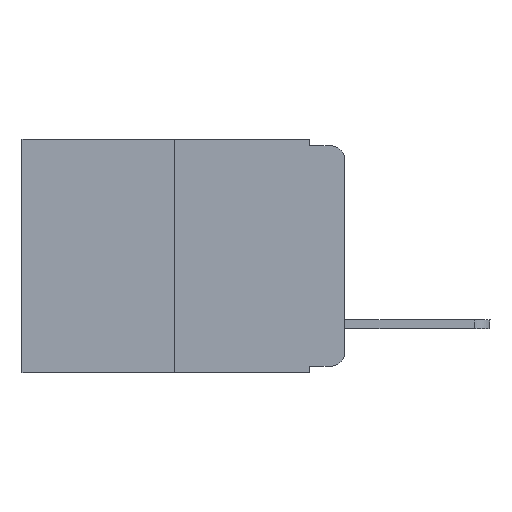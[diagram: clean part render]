
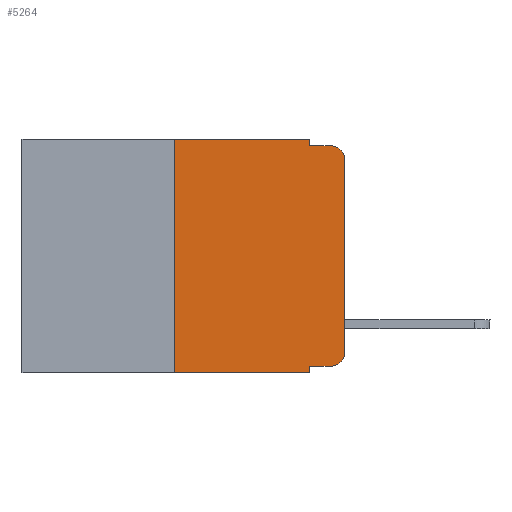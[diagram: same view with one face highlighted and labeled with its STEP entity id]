
A CAD part, left-side view. The second image highlights one B-rep face of the part: STEP entity #5264.
In plain terms, the highlighted planar face has unit normal (-1, 0, 0).
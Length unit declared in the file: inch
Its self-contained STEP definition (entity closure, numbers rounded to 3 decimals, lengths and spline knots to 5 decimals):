
#250 = EDGE_CURVE ( 'NONE', #9479, #11824, #8572, .T. ) ;
#260 = VECTOR ( 'NONE', #2099, 39.37008 ) ;
#417 = ORIENTED_EDGE ( 'NONE', *, *, #2067, .F. ) ;
#451 = EDGE_CURVE ( 'NONE', #14695, #15219, #6794, .T. ) ;
#776 = DIRECTION ( 'NONE',  ( 0., 0., -1. ) ) ;
#1366 = CARTESIAN_POINT ( 'NONE',  ( 0., 0.02, -0.01 ) ) ;
#1381 = EDGE_CURVE ( 'NONE', #6574, #12329, #13996, .T. ) ;
#1649 = LINE ( 'NONE', #4999, #11156 ) ;
#1793 = VECTOR ( 'NONE', #5993, 39.37008 ) ;
#2029 = CARTESIAN_POINT ( 'NONE',  ( 0., 0.051, 0. ) ) ;
#2041 = VECTOR ( 'NONE', #11379, 39.37008 ) ;
#2067 = EDGE_CURVE ( 'NONE', #7945, #11824, #14886, .T. ) ;
#2099 = DIRECTION ( 'NONE',  ( 0., 0., 1. ) ) ;
#2555 = VECTOR ( 'NONE', #5166, 39.37008 ) ;
#2570 = ORIENTED_EDGE ( 'NONE', *, *, #13722, .T. ) ;
#2808 = CARTESIAN_POINT ( 'NONE',  ( 0., 0.25, -0.343 ) ) ;
#2891 = CARTESIAN_POINT ( 'NONE',  ( 0., 0., 0. ) ) ;
#3054 = DIRECTION ( 'NONE',  ( 0., 0., 1. ) ) ;
#3152 = ORIENTED_EDGE ( 'NONE', *, *, #7505, .F. ) ;
#3263 = CARTESIAN_POINT ( 'NONE',  ( 0., 0.473, 0. ) ) ;
#3292 = CARTESIAN_POINT ( 'NONE',  ( 0., 0.051, -0.333 ) ) ;
#3336 = VERTEX_POINT ( 'NONE', #2808 ) ;
#3436 = ORIENTED_EDGE ( 'NONE', *, *, #4660, .F. ) ;
#3578 = AXIS2_PLACEMENT_3D ( 'NONE', #7578, #4042, #12323 ) ;
#3609 = CARTESIAN_POINT ( 'NONE',  ( 0., 0.02, -0.333 ) ) ;
#4042 = DIRECTION ( 'NONE',  ( -1., 0., 0. ) ) ;
#4388 = ORIENTED_EDGE ( 'NONE', *, *, #9475, .T. ) ;
#4435 = PLANE ( 'NONE',  #4990 ) ;
#4517 = LINE ( 'NONE', #5526, #260 ) ;
#4660 = EDGE_CURVE ( 'NONE', #15219, #7945, #6656, .T. ) ;
#4837 = CARTESIAN_POINT ( 'NONE',  ( 0., 0.25, 0. ) ) ;
#4990 = AXIS2_PLACEMENT_3D ( 'NONE', #3263, #12548, #776 ) ;
#4999 = CARTESIAN_POINT ( 'NONE',  ( 0., 0.051, 0. ) ) ;
#5076 = EDGE_LOOP ( 'NONE', ( #2570, #13152, #417, #3436, #9999, #10802, #4388, #3152, #5623, #9858 ) ) ;
#5166 = DIRECTION ( 'NONE',  ( 0., 0., -1. ) ) ;
#5264 = ADVANCED_FACE ( 'NONE', ( #11463 ), #4435, .F. ) ;
#5526 = CARTESIAN_POINT ( 'NONE',  ( 0., 0.25, 0. ) ) ;
#5623 = ORIENTED_EDGE ( 'NONE', *, *, #1381, .T. ) ;
#5993 = DIRECTION ( 'NONE',  ( 0., -1., 0. ) ) ;
#6017 = EDGE_CURVE ( 'NONE', #12329, #7464, #10867, .T. ) ;
#6271 = CARTESIAN_POINT ( 'NONE',  ( 0., 0.051, -0.343 ) ) ;
#6347 = DIRECTION ( 'NONE',  ( 0., 0., -1. ) ) ;
#6574 = VERTEX_POINT ( 'NONE', #7779 ) ;
#6656 = LINE ( 'NONE', #2029, #2555 ) ;
#6794 = LINE ( 'NONE', #8109, #12299 ) ;
#7464 = VERTEX_POINT ( 'NONE', #11172 ) ;
#7505 = EDGE_CURVE ( 'NONE', #6574, #13592, #1649, .T. ) ;
#7578 = CARTESIAN_POINT ( 'NONE',  ( 0., 0.02, -0.03 ) ) ;
#7779 = CARTESIAN_POINT ( 'NONE',  ( 0., 0.051, -0.333 ) ) ;
#7945 = VERTEX_POINT ( 'NONE', #8680 ) ;
#8058 = DIRECTION ( 'NONE',  ( 0., -1., 0. ) ) ;
#8109 = CARTESIAN_POINT ( 'NONE',  ( 0., 0.473, 0. ) ) ;
#8572 = CIRCLE ( 'NONE', #3578, 0.02 ) ;
#8680 = CARTESIAN_POINT ( 'NONE',  ( 0., 0.051, -0.01 ) ) ;
#8946 = CARTESIAN_POINT ( 'NONE',  ( 0., 0.02, -0.313 ) ) ;
#9306 = CARTESIAN_POINT ( 'NONE',  ( 0., 0.051, 0. ) ) ;
#9475 = EDGE_CURVE ( 'NONE', #3336, #13592, #11856, .T. ) ;
#9479 = VERTEX_POINT ( 'NONE', #10836 ) ;
#9858 = ORIENTED_EDGE ( 'NONE', *, *, #6017, .T. ) ;
#9999 = ORIENTED_EDGE ( 'NONE', *, *, #451, .F. ) ;
#10598 = DIRECTION ( 'NONE',  ( 0., -1., 0. ) ) ;
#10802 = ORIENTED_EDGE ( 'NONE', *, *, #14309, .F. ) ;
#10836 = CARTESIAN_POINT ( 'NONE',  ( 0., 0., -0.03 ) ) ;
#10867 = CIRCLE ( 'NONE', #14386, 0.02 ) ;
#11156 = VECTOR ( 'NONE', #6347, 39.37008 ) ;
#11172 = CARTESIAN_POINT ( 'NONE',  ( 0., 0., -0.313 ) ) ;
#11379 = DIRECTION ( 'NONE',  ( 0., -1., 0. ) ) ;
#11463 = FACE_OUTER_BOUND ( 'NONE', #5076, .T. ) ;
#11512 = DIRECTION ( 'NONE',  ( -1., 0., 0. ) ) ;
#11541 = VECTOR ( 'NONE', #8058, 39.37008 ) ;
#11592 = VECTOR ( 'NONE', #3054, 39.37008 ) ;
#11824 = VERTEX_POINT ( 'NONE', #1366 ) ;
#11856 = LINE ( 'NONE', #12949, #1793 ) ;
#12299 = VECTOR ( 'NONE', #10598, 39.37008 ) ;
#12323 = DIRECTION ( 'NONE',  ( 0., 0., -1. ) ) ;
#12329 = VERTEX_POINT ( 'NONE', #3609 ) ;
#12348 = LINE ( 'NONE', #2891, #11592 ) ;
#12532 = CARTESIAN_POINT ( 'NONE',  ( 0., 0.051, -0.01 ) ) ;
#12548 = DIRECTION ( 'NONE',  ( 1., 0., 0. ) ) ;
#12949 = CARTESIAN_POINT ( 'NONE',  ( 0., 0.473, -0.343 ) ) ;
#13152 = ORIENTED_EDGE ( 'NONE', *, *, #250, .T. ) ;
#13592 = VERTEX_POINT ( 'NONE', #6271 ) ;
#13722 = EDGE_CURVE ( 'NONE', #7464, #9479, #12348, .T. ) ;
#13996 = LINE ( 'NONE', #3292, #11541 ) ;
#14309 = EDGE_CURVE ( 'NONE', #3336, #14695, #4517, .T. ) ;
#14386 = AXIS2_PLACEMENT_3D ( 'NONE', #8946, #11512, #14864 ) ;
#14695 = VERTEX_POINT ( 'NONE', #4837 ) ;
#14864 = DIRECTION ( 'NONE',  ( 0., 0., -1. ) ) ;
#14886 = LINE ( 'NONE', #12532, #2041 ) ;
#15219 = VERTEX_POINT ( 'NONE', #9306 ) ;
